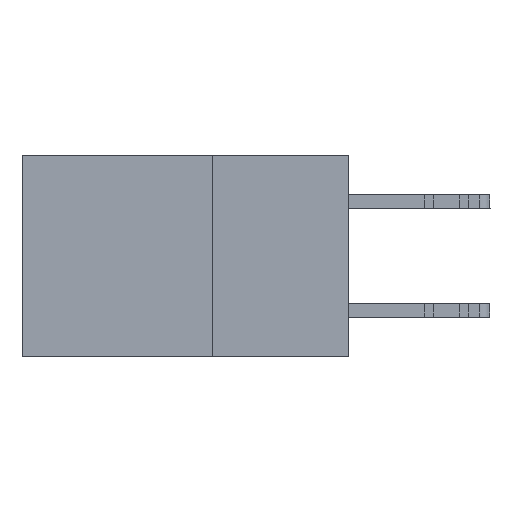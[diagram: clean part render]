
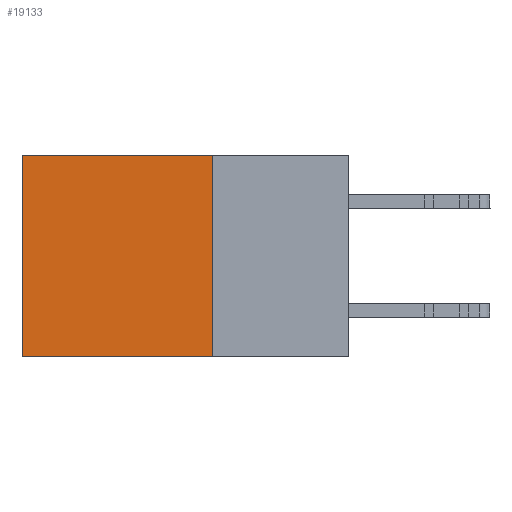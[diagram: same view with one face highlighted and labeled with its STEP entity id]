
A CAD part, left-side view. The second image highlights one B-rep face of the part: STEP entity #19133.
In plain terms, the highlighted planar face has unit normal (-1, 0, 0).
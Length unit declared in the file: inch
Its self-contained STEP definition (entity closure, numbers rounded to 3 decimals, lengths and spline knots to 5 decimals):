
#695 = EDGE_LOOP ( 'NONE', ( #17047, #3294, #13781, #16920 ) ) ;
#827 = CARTESIAN_POINT ( 'NONE',  ( 0.2615, 0.6, 0. ) ) ;
#3175 = DIRECTION ( 'NONE',  ( 0., 1., 0. ) ) ;
#3294 = ORIENTED_EDGE ( 'NONE', *, *, #25001, .F. ) ;
#3390 = DIRECTION ( 'NONE',  ( 1., 0., 0. ) ) ;
#3472 = CARTESIAN_POINT ( 'NONE',  ( 0.2615, 0.25, -0.37 ) ) ;
#3953 = EDGE_CURVE ( 'NONE', #20501, #24032, #12434, .T. ) ;
#4305 = CARTESIAN_POINT ( 'NONE',  ( 0.2615, 0.25, -0.37 ) ) ;
#5874 = CARTESIAN_POINT ( 'NONE',  ( 0.2615, 0.6, -0.37 ) ) ;
#6519 = LINE ( 'NONE', #22136, #6823 ) ;
#6823 = VECTOR ( 'NONE', #14272, 39.37008 ) ;
#7152 = VECTOR ( 'NONE', #8488, 39.37008 ) ;
#7319 = CARTESIAN_POINT ( 'NONE',  ( 0.2615, 0.25, -0.37 ) ) ;
#7429 = DIRECTION ( 'NONE',  ( 0., 0., -1. ) ) ;
#8488 = DIRECTION ( 'NONE',  ( 0., 0., -1. ) ) ;
#8628 = CARTESIAN_POINT ( 'NONE',  ( 0.2615, 0.25, 0. ) ) ;
#9202 = CARTESIAN_POINT ( 'NONE',  ( 0.2615, 0.25, 0. ) ) ;
#9332 = PLANE ( 'NONE',  #15743 ) ;
#11622 = VECTOR ( 'NONE', #3175, 39.37008 ) ;
#12267 = EDGE_CURVE ( 'NONE', #16641, #14961, #12902, .T. ) ;
#12434 = LINE ( 'NONE', #4305, #7152 ) ;
#12902 = LINE ( 'NONE', #24837, #13548 ) ;
#13548 = VECTOR ( 'NONE', #7429, 39.37008 ) ;
#13781 = ORIENTED_EDGE ( 'NONE', *, *, #3953, .F. ) ;
#14272 = DIRECTION ( 'NONE',  ( 0., 1., 0. ) ) ;
#14961 = VERTEX_POINT ( 'NONE', #5874 ) ;
#15743 = AXIS2_PLACEMENT_3D ( 'NONE', #7319, #3390, #22939 ) ;
#16641 = VERTEX_POINT ( 'NONE', #827 ) ;
#16920 = ORIENTED_EDGE ( 'NONE', *, *, #17076, .T. ) ;
#17047 = ORIENTED_EDGE ( 'NONE', *, *, #12267, .T. ) ;
#17076 = EDGE_CURVE ( 'NONE', #20501, #16641, #20564, .T. ) ;
#19133 = ADVANCED_FACE ( 'NONE', ( #20650 ), #9332, .F. ) ;
#20501 = VERTEX_POINT ( 'NONE', #9202 ) ;
#20564 = LINE ( 'NONE', #8628, #11622 ) ;
#20650 = FACE_OUTER_BOUND ( 'NONE', #695, .T. ) ;
#22136 = CARTESIAN_POINT ( 'NONE',  ( 0.2615, 0.25, -0.37 ) ) ;
#22939 = DIRECTION ( 'NONE',  ( 0., 0., -1. ) ) ;
#24032 = VERTEX_POINT ( 'NONE', #3472 ) ;
#24837 = CARTESIAN_POINT ( 'NONE',  ( 0.2615, 0.6, -0.37 ) ) ;
#25001 = EDGE_CURVE ( 'NONE', #24032, #14961, #6519, .T. ) ;
